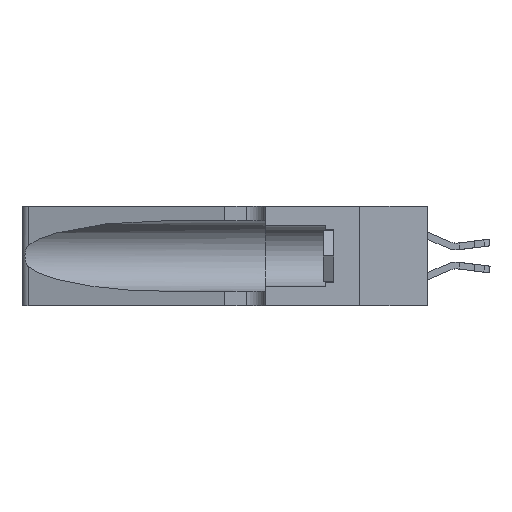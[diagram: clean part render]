
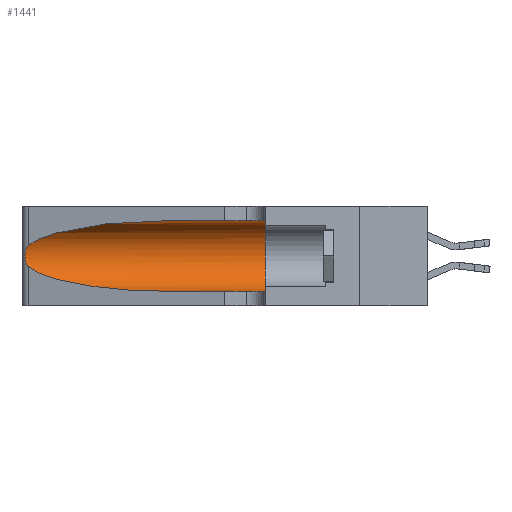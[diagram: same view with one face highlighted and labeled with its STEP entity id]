
A CAD part, left-side view. The second image highlights one B-rep face of the part: STEP entity #1441.
In plain terms, the highlighted cylindrical face has radius 3.308 mm (diameter 6.617 mm), a partial arc.
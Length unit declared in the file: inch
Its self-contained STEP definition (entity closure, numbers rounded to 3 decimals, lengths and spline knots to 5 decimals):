
#83 = AXIS2_PLACEMENT_3D ( 'NONE', #17801, #8406, #19355 ) ;
#365 =( BOUNDED_CURVE ( )  B_SPLINE_CURVE ( 3, ( #10899, #1433, #7881, #18860 ),
 .UNSPECIFIED., .F., .F. ) 
 B_SPLINE_CURVE_WITH_KNOTS ( ( 4, 4 ),
 ( 1.5708, 2.84003 ),
 .UNSPECIFIED. ) 
 CURVE ( )  GEOMETRIC_REPRESENTATION_ITEM ( )  RATIONAL_B_SPLINE_CURVE ( ( 1., 0.87, 0.87, 1. ) ) 
 REPRESENTATION_ITEM ( '' )  );
#542 = VERTEX_POINT ( 'NONE', #8216 ) ;
#612 = DIRECTION ( 'NONE',  ( 0., -1., 0. ) ) ;
#933 = B_SPLINE_CURVE_WITH_KNOTS ( 'NONE', 3,
 ( #19976, #9029, #18421, #1031, #12158, #2694, #13731, #4297, #15318, #5893, #16916, #7498, #18488, #9098 ),
 .UNSPECIFIED., .F., .F.,
 ( 4, 2, 2, 2, 2, 2, 4 ),
 ( 0., 0.00027, 0.00053, 0.00107, 0.0016, 0.00187, 0.00214 ),
 .UNSPECIFIED. ) ;
#1031 = CARTESIAN_POINT ( 'NONE',  ( 0.25787, 1.23484, 0.2124 ) ) ;
#1433 = CARTESIAN_POINT ( 'NONE',  ( 0.18966, 0.96281, 0.31525 ) ) ;
#1441 = ADVANCED_FACE ( 'NONE', ( #20175 ), #7665, .F. ) ;
#1745 = ORIENTED_EDGE ( 'NONE', *, *, #14347, .T. ) ;
#1912 = ORIENTED_EDGE ( 'NONE', *, *, #7907, .T. ) ;
#2244 = CARTESIAN_POINT ( 'NONE',  ( 0.1305, 1.61858, 0.185 ) ) ;
#2346 = LINE ( 'NONE', #11759, #14943 ) ;
#2694 = CARTESIAN_POINT ( 'NONE',  ( 0.26018, 1.23835, 0.19895 ) ) ;
#2923 = AXIS2_PLACEMENT_3D ( 'NONE', #2244, #10643, #10703 ) ;
#3497 = VERTEX_POINT ( 'NONE', #7007 ) ;
#3537 =( BOUNDED_CURVE ( )  B_SPLINE_CURVE ( 3, ( #17079, #7675, #18653, #9266 ),
 .UNSPECIFIED., .F., .F. ) 
 B_SPLINE_CURVE_WITH_KNOTS ( ( 4, 4 ),
 ( 3.44316, 4.71239 ),
 .UNSPECIFIED. ) 
 CURVE ( )  GEOMETRIC_REPRESENTATION_ITEM ( )  RATIONAL_B_SPLINE_CURVE ( ( 1., 0.87, 0.87, 1. ) ) 
 REPRESENTATION_ITEM ( '' )  );
#3612 = CARTESIAN_POINT ( 'NONE',  ( 0.25487, 1.22718, 0.22369 ) ) ;
#4297 = CARTESIAN_POINT ( 'NONE',  ( 0.26075, 1.23896, 0.178 ) ) ;
#5363 = EDGE_CURVE ( 'NONE', #8681, #20395, #933, .T. ) ;
#5526 = EDGE_LOOP ( 'NONE', ( #1912, #5625, #8835, #1745, #7262, #9641 ) ) ;
#5625 = ORIENTED_EDGE ( 'NONE', *, *, #5363, .T. ) ;
#5893 = CARTESIAN_POINT ( 'NONE',  ( 0.25856, 1.23593, 0.16098 ) ) ;
#6454 = VERTEX_POINT ( 'NONE', #16737 ) ;
#6889 = LINE ( 'NONE', #11619, #18449 ) ;
#6903 = CIRCLE ( 'NONE', #83, 0.13025 ) ;
#7007 = CARTESIAN_POINT ( 'NONE',  ( 0.1305, 0.72297, 0.05475 ) ) ;
#7262 = ORIENTED_EDGE ( 'NONE', *, *, #12763, .F. ) ;
#7498 = CARTESIAN_POINT ( 'NONE',  ( 0.25639, 1.23186, 0.15144 ) ) ;
#7665 = CYLINDRICAL_SURFACE ( 'NONE', #2923, 0.13025 ) ;
#7675 = CARTESIAN_POINT ( 'NONE',  ( 0.2373, 1.15595, 0.08982 ) ) ;
#7726 = VERTEX_POINT ( 'NONE', #10557 ) ;
#7881 = CARTESIAN_POINT ( 'NONE',  ( 0.2373, 1.15595, 0.28018 ) ) ;
#7907 = EDGE_CURVE ( 'NONE', #6454, #8681, #365, .T. ) ;
#8207 = EDGE_CURVE ( 'NONE', #6454, #542, #6889, .T. ) ;
#8216 = CARTESIAN_POINT ( 'NONE',  ( 0.1305, 0.35, 0.31525 ) ) ;
#8406 = DIRECTION ( 'NONE',  ( 0., 1., 0. ) ) ;
#8681 = VERTEX_POINT ( 'NONE', #3612 ) ;
#8835 = ORIENTED_EDGE ( 'NONE', *, *, #9658, .T. ) ;
#9029 = CARTESIAN_POINT ( 'NONE',  ( 0.25555, 1.22994, 0.2215 ) ) ;
#9098 = CARTESIAN_POINT ( 'NONE',  ( 0.25487, 1.22718, 0.14631 ) ) ;
#9266 = CARTESIAN_POINT ( 'NONE',  ( 0.1305, 0.72297, 0.05475 ) ) ;
#9641 = ORIENTED_EDGE ( 'NONE', *, *, #8207, .F. ) ;
#9658 = EDGE_CURVE ( 'NONE', #20395, #3497, #3537, .T. ) ;
#9995 = DIRECTION ( 'NONE',  ( 0., -1., 0. ) ) ;
#10557 = CARTESIAN_POINT ( 'NONE',  ( 0.1305, 0.35, 0.05475 ) ) ;
#10643 = DIRECTION ( 'NONE',  ( 0., -1., 0. ) ) ;
#10703 = DIRECTION ( 'NONE',  ( 0., 0., -1. ) ) ;
#10899 = CARTESIAN_POINT ( 'NONE',  ( 0.1305, 0.72297, 0.31525 ) ) ;
#11619 = CARTESIAN_POINT ( 'NONE',  ( 0.1305, 1.61858, 0.31525 ) ) ;
#11759 = CARTESIAN_POINT ( 'NONE',  ( 0.1305, 1.61858, 0.05475 ) ) ;
#12158 = CARTESIAN_POINT ( 'NONE',  ( 0.25854, 1.2359, 0.20912 ) ) ;
#12694 = CARTESIAN_POINT ( 'NONE',  ( 0.25487, 1.22718, 0.14631 ) ) ;
#12763 = EDGE_CURVE ( 'NONE', #542, #7726, #6903, .T. ) ;
#13731 = CARTESIAN_POINT ( 'NONE',  ( 0.26075, 1.23896, 0.19203 ) ) ;
#14347 = EDGE_CURVE ( 'NONE', #3497, #7726, #2346, .T. ) ;
#14943 = VECTOR ( 'NONE', #612, 39.37008 ) ;
#15318 = CARTESIAN_POINT ( 'NONE',  ( 0.26017, 1.23833, 0.17102 ) ) ;
#16737 = CARTESIAN_POINT ( 'NONE',  ( 0.1305, 0.72297, 0.31525 ) ) ;
#16916 = CARTESIAN_POINT ( 'NONE',  ( 0.25789, 1.23486, 0.15765 ) ) ;
#17079 = CARTESIAN_POINT ( 'NONE',  ( 0.25487, 1.22718, 0.14631 ) ) ;
#17801 = CARTESIAN_POINT ( 'NONE',  ( 0.1305, 0.35, 0.185 ) ) ;
#18421 = CARTESIAN_POINT ( 'NONE',  ( 0.25639, 1.23184, 0.21858 ) ) ;
#18449 = VECTOR ( 'NONE', #9995, 39.37008 ) ;
#18488 = CARTESIAN_POINT ( 'NONE',  ( 0.25555, 1.22993, 0.14849 ) ) ;
#18653 = CARTESIAN_POINT ( 'NONE',  ( 0.18966, 0.96281, 0.05475 ) ) ;
#18860 = CARTESIAN_POINT ( 'NONE',  ( 0.25487, 1.22718, 0.22369 ) ) ;
#19355 = DIRECTION ( 'NONE',  ( 0., 0., 1. ) ) ;
#19976 = CARTESIAN_POINT ( 'NONE',  ( 0.25487, 1.22718, 0.22369 ) ) ;
#20175 = FACE_OUTER_BOUND ( 'NONE', #5526, .T. ) ;
#20395 = VERTEX_POINT ( 'NONE', #12694 ) ;
